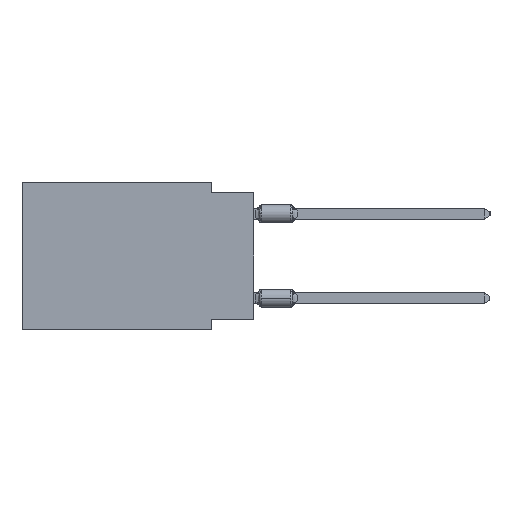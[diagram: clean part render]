
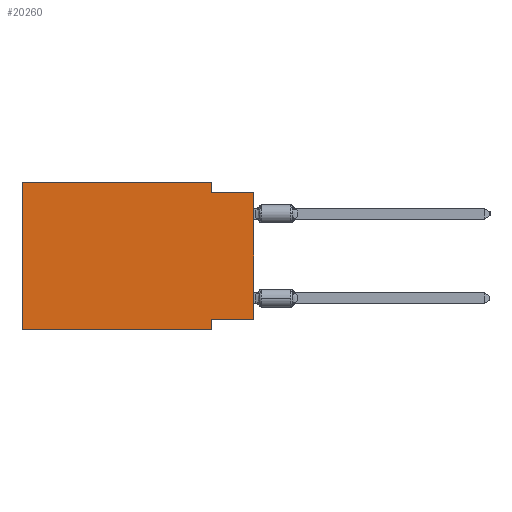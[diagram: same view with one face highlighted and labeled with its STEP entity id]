
A CAD part, left-side view. The second image highlights one B-rep face of the part: STEP entity #20260.
In plain terms, the highlighted planar face has unit normal (-1, 0, 0).
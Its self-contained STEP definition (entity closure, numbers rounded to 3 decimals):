
#104 = CARTESIAN_POINT ( 'NONE',  ( 0., 13.97, 0. ) ) ;
#549 = CARTESIAN_POINT ( 'NONE',  ( 0., 2.54, -0.635 ) ) ;
#1887 = ORIENTED_EDGE ( 'NONE', *, *, #19232, .F. ) ;
#2135 = DIRECTION ( 'NONE',  ( 0., 0., -1. ) ) ;
#3270 = VERTEX_POINT ( 'NONE', #29587 ) ;
#3656 = DIRECTION ( 'NONE',  ( 0., 0., -1. ) ) ;
#5311 = DIRECTION ( 'NONE',  ( 0., 1., 0. ) ) ;
#5528 = EDGE_CURVE ( 'NONE', #19157, #20591, #9961, .T. ) ;
#5883 = VECTOR ( 'NONE', #6046, 1000. ) ;
#6046 = DIRECTION ( 'NONE',  ( 0., -1., 0. ) ) ;
#6172 = CARTESIAN_POINT ( 'NONE',  ( 0., 13.97, -8.89 ) ) ;
#7067 = DIRECTION ( 'NONE',  ( 0., 0., 1. ) ) ;
#7821 = ORIENTED_EDGE ( 'NONE', *, *, #32889, .F. ) ;
#8241 = LINE ( 'NONE', #25518, #36680 ) ;
#8478 = DIRECTION ( 'NONE',  ( 0., 0., -1. ) ) ;
#8935 = LINE ( 'NONE', #35657, #39153 ) ;
#9101 = FACE_OUTER_BOUND ( 'NONE', #22122, .T. ) ;
#9826 = VECTOR ( 'NONE', #8478, 1000. ) ;
#9961 = LINE ( 'NONE', #23640, #33255 ) ;
#10011 = CARTESIAN_POINT ( 'NONE',  ( 0., 2.54, -8.255 ) ) ;
#10528 = AXIS2_PLACEMENT_3D ( 'NONE', #43220, #13369, #2135 ) ;
#11175 = ORIENTED_EDGE ( 'NONE', *, *, #32462, .F. ) ;
#12291 = LINE ( 'NONE', #22382, #9826 ) ;
#12408 = CARTESIAN_POINT ( 'NONE',  ( 0., 0., -0.635 ) ) ;
#12693 = CARTESIAN_POINT ( 'NONE',  ( 0., 0., -8.255 ) ) ;
#13369 = DIRECTION ( 'NONE',  ( 1., 0., 0. ) ) ;
#14744 = EDGE_CURVE ( 'NONE', #26753, #3270, #15915, .T. ) ;
#15522 = ORIENTED_EDGE ( 'NONE', *, *, #27459, .F. ) ;
#15915 = LINE ( 'NONE', #43562, #5883 ) ;
#16579 = ORIENTED_EDGE ( 'NONE', *, *, #5528, .F. ) ;
#16936 = DIRECTION ( 'NONE',  ( 0., -1., 0. ) ) ;
#17190 = ORIENTED_EDGE ( 'NONE', *, *, #19669, .F. ) ;
#19009 = VERTEX_POINT ( 'NONE', #12693 ) ;
#19157 = VERTEX_POINT ( 'NONE', #549 ) ;
#19232 = EDGE_CURVE ( 'NONE', #26753, #29031, #30854, .T. ) ;
#19669 = EDGE_CURVE ( 'NONE', #29031, #31628, #8935, .T. ) ;
#20260 = ADVANCED_FACE ( 'NONE', ( #9101 ), #26374, .F. ) ;
#20591 = VERTEX_POINT ( 'NONE', #12408 ) ;
#21249 = ORIENTED_EDGE ( 'NONE', *, *, #33835, .T. ) ;
#21917 = VERTEX_POINT ( 'NONE', #10011 ) ;
#22122 = EDGE_LOOP ( 'NONE', ( #21249, #16579, #15522, #17190, #1887, #34902, #11175, #7821 ) ) ;
#22382 = CARTESIAN_POINT ( 'NONE',  ( 0., 2.54, 0. ) ) ;
#23640 = CARTESIAN_POINT ( 'NONE',  ( 0., 0., -0.635 ) ) ;
#23763 = LINE ( 'NONE', #31548, #31702 ) ;
#24437 = VECTOR ( 'NONE', #3656, 1000. ) ;
#25518 = CARTESIAN_POINT ( 'NONE',  ( 0., 0., -8.255 ) ) ;
#26374 = PLANE ( 'NONE',  #10528 ) ;
#26753 = VERTEX_POINT ( 'NONE', #6172 ) ;
#27459 = EDGE_CURVE ( 'NONE', #31628, #19157, #12291, .T. ) ;
#29031 = VERTEX_POINT ( 'NONE', #39861 ) ;
#29096 = CARTESIAN_POINT ( 'NONE',  ( 0., 2.54, 0. ) ) ;
#29587 = CARTESIAN_POINT ( 'NONE',  ( 0., 2.54, -8.89 ) ) ;
#30059 = DIRECTION ( 'NONE',  ( 0., 0., 1. ) ) ;
#30854 = LINE ( 'NONE', #104, #36271 ) ;
#31548 = CARTESIAN_POINT ( 'NONE',  ( 0., 0., 0. ) ) ;
#31628 = VERTEX_POINT ( 'NONE', #29096 ) ;
#31702 = VECTOR ( 'NONE', #30059, 1000. ) ;
#32278 = DIRECTION ( 'NONE',  ( 0., -1., 0. ) ) ;
#32462 = EDGE_CURVE ( 'NONE', #21917, #3270, #41395, .T. ) ;
#32889 = EDGE_CURVE ( 'NONE', #19009, #21917, #8241, .T. ) ;
#33255 = VECTOR ( 'NONE', #16936, 1000. ) ;
#33835 = EDGE_CURVE ( 'NONE', #19009, #20591, #23763, .T. ) ;
#34217 = CARTESIAN_POINT ( 'NONE',  ( 0., 2.54, -8.89 ) ) ;
#34902 = ORIENTED_EDGE ( 'NONE', *, *, #14744, .T. ) ;
#35657 = CARTESIAN_POINT ( 'NONE',  ( 0., 13.97, 0. ) ) ;
#36271 = VECTOR ( 'NONE', #7067, 1000. ) ;
#36680 = VECTOR ( 'NONE', #5311, 1000. ) ;
#39153 = VECTOR ( 'NONE', #32278, 1000. ) ;
#39861 = CARTESIAN_POINT ( 'NONE',  ( 0., 13.97, 0. ) ) ;
#41395 = LINE ( 'NONE', #34217, #24437 ) ;
#43220 = CARTESIAN_POINT ( 'NONE',  ( 0., 13.97, 0. ) ) ;
#43562 = CARTESIAN_POINT ( 'NONE',  ( 0., 13.97, -8.89 ) ) ;
